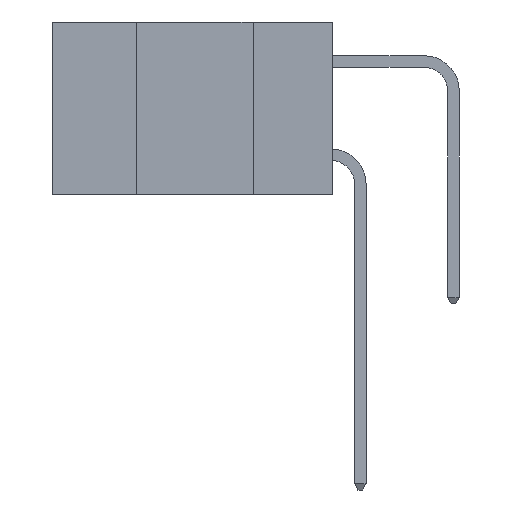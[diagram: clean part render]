
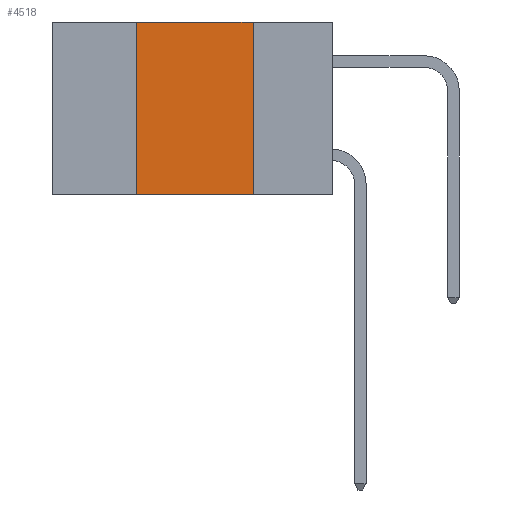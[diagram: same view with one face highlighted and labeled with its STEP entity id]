
A CAD part, left-side view. The second image highlights one B-rep face of the part: STEP entity #4518.
In plain terms, the highlighted planar face has unit normal (-1, 0, 0).
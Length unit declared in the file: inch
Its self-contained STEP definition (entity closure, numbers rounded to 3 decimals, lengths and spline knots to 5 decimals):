
#276 = CARTESIAN_POINT ( 'NONE',  ( 0., 0.6, 0. ) ) ;
#289 = LINE ( 'NONE', #20880, #17077 ) ;
#529 = ORIENTED_EDGE ( 'NONE', *, *, #9497, .F. ) ;
#1463 = CARTESIAN_POINT ( 'NONE',  ( 0., 0.17, -0.37 ) ) ;
#1707 = LINE ( 'NONE', #6986, #18394 ) ;
#1985 = PLANE ( 'NONE',  #3568 ) ;
#3163 = ORIENTED_EDGE ( 'NONE', *, *, #8377, .T. ) ;
#3568 = AXIS2_PLACEMENT_3D ( 'NONE', #276, #13361, #3655 ) ;
#3655 = DIRECTION ( 'NONE',  ( 0., 0., -1. ) ) ;
#4518 = ADVANCED_FACE ( 'NONE', ( #17667 ), #1985, .F. ) ;
#4857 = CARTESIAN_POINT ( 'NONE',  ( 0., 0.17, 0. ) ) ;
#5038 = EDGE_LOOP ( 'NONE', ( #12030, #5354, #529, #3163 ) ) ;
#5354 = ORIENTED_EDGE ( 'NONE', *, *, #10609, .F. ) ;
#6986 = CARTESIAN_POINT ( 'NONE',  ( 0., 0.17, -0.37 ) ) ;
#7662 = VECTOR ( 'NONE', #7977, 39.37008 ) ;
#7880 = CARTESIAN_POINT ( 'NONE',  ( 0., 0.6, 0. ) ) ;
#7977 = DIRECTION ( 'NONE',  ( 0., 0., 1. ) ) ;
#8377 = EDGE_CURVE ( 'NONE', #13566, #17661, #289, .T. ) ;
#8649 = LINE ( 'NONE', #7880, #20872 ) ;
#9497 = EDGE_CURVE ( 'NONE', #13566, #11401, #11494, .T. ) ;
#9555 = DIRECTION ( 'NONE',  ( 0., -1., 0. ) ) ;
#10609 = EDGE_CURVE ( 'NONE', #11401, #20046, #8649, .T. ) ;
#11401 = VERTEX_POINT ( 'NONE', #16283 ) ;
#11494 = LINE ( 'NONE', #19214, #7662 ) ;
#12030 = ORIENTED_EDGE ( 'NONE', *, *, #12758, .F. ) ;
#12758 = EDGE_CURVE ( 'NONE', #20046, #17661, #1707, .T. ) ;
#13361 = DIRECTION ( 'NONE',  ( 1., 0., 0. ) ) ;
#13566 = VERTEX_POINT ( 'NONE', #16513 ) ;
#16235 = DIRECTION ( 'NONE',  ( 0., -1., 0. ) ) ;
#16283 = CARTESIAN_POINT ( 'NONE',  ( 0., 0.42, 0. ) ) ;
#16513 = CARTESIAN_POINT ( 'NONE',  ( 0., 0.42, -0.37 ) ) ;
#17077 = VECTOR ( 'NONE', #16235, 39.37008 ) ;
#17661 = VERTEX_POINT ( 'NONE', #1463 ) ;
#17667 = FACE_OUTER_BOUND ( 'NONE', #5038, .T. ) ;
#18394 = VECTOR ( 'NONE', #19803, 39.37008 ) ;
#19214 = CARTESIAN_POINT ( 'NONE',  ( 0., 0.42, -0.37 ) ) ;
#19803 = DIRECTION ( 'NONE',  ( 0., 0., -1. ) ) ;
#20046 = VERTEX_POINT ( 'NONE', #4857 ) ;
#20872 = VECTOR ( 'NONE', #9555, 39.37008 ) ;
#20880 = CARTESIAN_POINT ( 'NONE',  ( 0., 0.6, -0.37 ) ) ;
